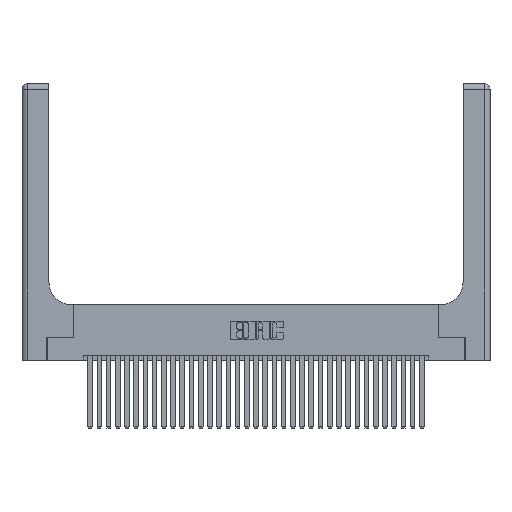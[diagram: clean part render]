
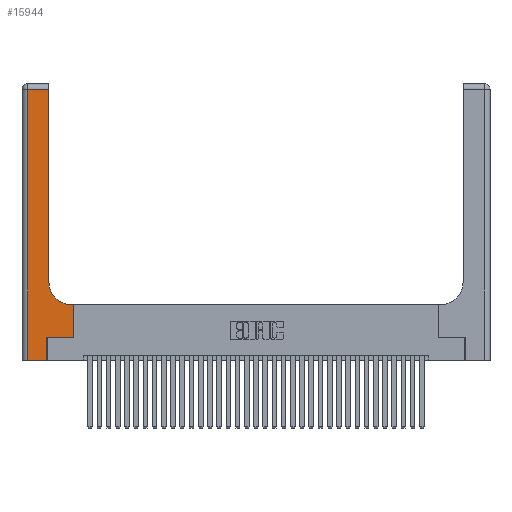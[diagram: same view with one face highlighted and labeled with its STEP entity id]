
A CAD part, top view. The second image highlights one B-rep face of the part: STEP entity #15944.
In plain terms, the highlighted planar face has unit normal (0, 0, 1).
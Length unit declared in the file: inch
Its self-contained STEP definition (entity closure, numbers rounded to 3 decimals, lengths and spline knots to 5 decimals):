
#257 = ORIENTED_EDGE ( 'NONE', *, *, #12177, .T. ) ;
#294 = VECTOR ( 'NONE', #10966, 39.37008 ) ;
#862 = VERTEX_POINT ( 'NONE', #18402 ) ;
#1392 = CARTESIAN_POINT ( 'NONE',  ( 0.2915, 2.94, 0.37 ) ) ;
#1593 = EDGE_CURVE ( 'NONE', #862, #10982, #28857, .T. ) ;
#1671 = CARTESIAN_POINT ( 'NONE',  ( 0.2915, 3., 0.37 ) ) ;
#1725 = EDGE_CURVE ( 'NONE', #23955, #20103, #3294, .T. ) ;
#2000 = CARTESIAN_POINT ( 'NONE',  ( 0.269, 0., 0.37 ) ) ;
#2098 = AXIS2_PLACEMENT_3D ( 'NONE', #29874, #13901, #32551 ) ;
#3294 = LINE ( 'NONE', #30072, #30919 ) ;
#3412 = DIRECTION ( 'NONE',  ( -1., 0., 0. ) ) ;
#3479 = LINE ( 'NONE', #21458, #16913 ) ;
#3863 = EDGE_CURVE ( 'NONE', #10982, #22390, #16632, .T. ) ;
#4230 = VERTEX_POINT ( 'NONE', #32828 ) ;
#4476 = PLANE ( 'NONE',  #21514 ) ;
#5406 = ORIENTED_EDGE ( 'NONE', *, *, #23309, .T. ) ;
#5942 = EDGE_CURVE ( 'NONE', #18663, #862, #3479, .T. ) ;
#5959 = VECTOR ( 'NONE', #29473, 39.37008 ) ;
#7165 = DIRECTION ( 'NONE',  ( -1., 0., 0. ) ) ;
#8120 = DIRECTION ( 'NONE',  ( 1., 0., 0. ) ) ;
#8554 = CARTESIAN_POINT ( 'NONE',  ( 0.5585, 0.6, 0.37 ) ) ;
#9551 = VECTOR ( 'NONE', #28909, 39.37008 ) ;
#10966 = DIRECTION ( 'NONE',  ( 0., 1., 0. ) ) ;
#10982 = VERTEX_POINT ( 'NONE', #8554 ) ;
#11492 = LINE ( 'NONE', #2000, #31935 ) ;
#12177 = EDGE_CURVE ( 'NONE', #20626, #4230, #13095, .T. ) ;
#13095 = LINE ( 'NONE', #29360, #5959 ) ;
#13237 = VERTEX_POINT ( 'NONE', #31233 ) ;
#13364 = CARTESIAN_POINT ( 'NONE',  ( 0.06, 3., 0.37 ) ) ;
#13763 = EDGE_LOOP ( 'NONE', ( #19224, #33386, #20062, #257, #14634, #28812, #16272, #18822, #5406 ) ) ;
#13901 = DIRECTION ( 'NONE',  ( 0., 0., -1. ) ) ;
#13991 = CIRCLE ( 'NONE', #2098, 0.25 ) ;
#14634 = ORIENTED_EDGE ( 'NONE', *, *, #24095, .T. ) ;
#14820 = CARTESIAN_POINT ( 'NONE',  ( 0.5415, 0.6, 0.37 ) ) ;
#15347 = CARTESIAN_POINT ( 'NONE',  ( 0.06, 0., 0.37 ) ) ;
#15395 = CARTESIAN_POINT ( 'NONE',  ( 0.2915, 0.6, 0.37 ) ) ;
#15944 = ADVANCED_FACE ( 'NONE', ( #29112 ), #4476, .F. ) ;
#16272 = ORIENTED_EDGE ( 'NONE', *, *, #1593, .T. ) ;
#16632 = LINE ( 'NONE', #15395, #9551 ) ;
#16913 = VECTOR ( 'NONE', #8120, 39.37008 ) ;
#17954 = EDGE_CURVE ( 'NONE', #20103, #20626, #25682, .T. ) ;
#18402 = CARTESIAN_POINT ( 'NONE',  ( 0.5585, 0.25, 0.37 ) ) ;
#18567 = VECTOR ( 'NONE', #29442, 39.37008 ) ;
#18663 = VERTEX_POINT ( 'NONE', #32531 ) ;
#18822 = ORIENTED_EDGE ( 'NONE', *, *, #3863, .T. ) ;
#19224 = ORIENTED_EDGE ( 'NONE', *, *, #23650, .T. ) ;
#20062 = ORIENTED_EDGE ( 'NONE', *, *, #17954, .T. ) ;
#20103 = VERTEX_POINT ( 'NONE', #30121 ) ;
#20626 = VERTEX_POINT ( 'NONE', #15347 ) ;
#21458 = CARTESIAN_POINT ( 'NONE',  ( 0.269, 0.25, 0.37 ) ) ;
#21514 = AXIS2_PLACEMENT_3D ( 'NONE', #23072, #23187, #7165 ) ;
#22390 = VERTEX_POINT ( 'NONE', #14820 ) ;
#23072 = CARTESIAN_POINT ( 'NONE',  ( 0., 3., 0.37 ) ) ;
#23187 = DIRECTION ( 'NONE',  ( 0., 0., -1. ) ) ;
#23309 = EDGE_CURVE ( 'NONE', #22390, #13237, #13991, .T. ) ;
#23650 = EDGE_CURVE ( 'NONE', #13237, #23955, #32793, .T. ) ;
#23955 = VERTEX_POINT ( 'NONE', #1392 ) ;
#24095 = EDGE_CURVE ( 'NONE', #4230, #18663, #11492, .T. ) ;
#24282 = CARTESIAN_POINT ( 'NONE',  ( 0.5585, 0.25, 0.37 ) ) ;
#25682 = LINE ( 'NONE', #13364, #18567 ) ;
#26575 = VECTOR ( 'NONE', #32174, 39.37008 ) ;
#28812 = ORIENTED_EDGE ( 'NONE', *, *, #5942, .T. ) ;
#28857 = LINE ( 'NONE', #24282, #294 ) ;
#28909 = DIRECTION ( 'NONE',  ( -1., 0., 0. ) ) ;
#29112 = FACE_OUTER_BOUND ( 'NONE', #13763, .T. ) ;
#29360 = CARTESIAN_POINT ( 'NONE',  ( 0., 0., 0.37 ) ) ;
#29442 = DIRECTION ( 'NONE',  ( 0., -1., 0. ) ) ;
#29473 = DIRECTION ( 'NONE',  ( 1., 0., 0. ) ) ;
#29874 = CARTESIAN_POINT ( 'NONE',  ( 0.5415, 0.85, 0.37 ) ) ;
#30072 = CARTESIAN_POINT ( 'NONE',  ( 0., 2.94, 0.37 ) ) ;
#30121 = CARTESIAN_POINT ( 'NONE',  ( 0.06, 2.94, 0.37 ) ) ;
#30919 = VECTOR ( 'NONE', #3412, 39.37008 ) ;
#31233 = CARTESIAN_POINT ( 'NONE',  ( 0.2915, 0.85, 0.37 ) ) ;
#31236 = DIRECTION ( 'NONE',  ( 0., 1., 0. ) ) ;
#31935 = VECTOR ( 'NONE', #31236, 39.37008 ) ;
#32174 = DIRECTION ( 'NONE',  ( 0., 1., 0. ) ) ;
#32531 = CARTESIAN_POINT ( 'NONE',  ( 0.269, 0.25, 0.37 ) ) ;
#32551 = DIRECTION ( 'NONE',  ( 1., 0., 0. ) ) ;
#32793 = LINE ( 'NONE', #1671, #26575 ) ;
#32828 = CARTESIAN_POINT ( 'NONE',  ( 0.269, 0., 0.37 ) ) ;
#33386 = ORIENTED_EDGE ( 'NONE', *, *, #1725, .T. ) ;
